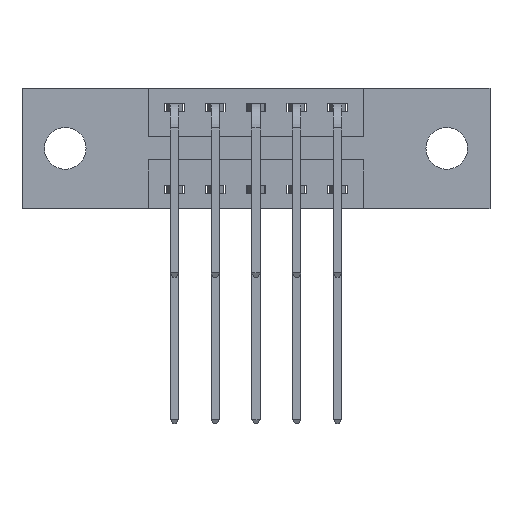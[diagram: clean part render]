
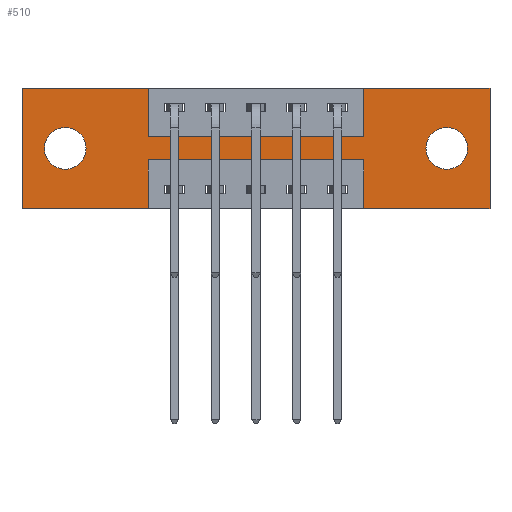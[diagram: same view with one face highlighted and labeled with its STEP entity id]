
A CAD part, front view. The second image highlights one B-rep face of the part: STEP entity #510.
In plain terms, the highlighted planar face has unit normal (0, -1, 0).
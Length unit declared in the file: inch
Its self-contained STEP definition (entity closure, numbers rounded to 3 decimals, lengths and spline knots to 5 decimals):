
#26 = LINE ( 'NONE', #8358, #9534 ) ;
#68 = VECTOR ( 'NONE', #4947, 39.37008 ) ;
#191 = LINE ( 'NONE', #3979, #1855 ) ;
#218 = VECTOR ( 'NONE', #2254, 39.37008 ) ;
#464 = ORIENTED_EDGE ( 'NONE', *, *, #4094, .T. ) ;
#473 = AXIS2_PLACEMENT_3D ( 'NONE', #3910, #2946, #4568 ) ;
#510 = ADVANCED_FACE ( 'NONE', ( #6806, #5420, #1509 ), #10048, .T. ) ;
#543 = CARTESIAN_POINT ( 'NONE',  ( 0., 0., 0. ) ) ;
#584 = VERTEX_POINT ( 'NONE', #8944 ) ;
#598 = ORIENTED_EDGE ( 'NONE', *, *, #5182, .F. ) ;
#751 = DIRECTION ( 'NONE',  ( 0., 0., 1. ) ) ;
#827 = DIRECTION ( 'NONE',  ( -1., 0., 0. ) ) ;
#832 = ORIENTED_EDGE ( 'NONE', *, *, #1442, .F. ) ;
#926 = EDGE_CURVE ( 'NONE', #9453, #1668, #6404, .T. ) ;
#937 = VERTEX_POINT ( 'NONE', #5608 ) ;
#1012 = CARTESIAN_POINT ( 'NONE',  ( 0., 0., -0.37 ) ) ;
#1016 = AXIS2_PLACEMENT_3D ( 'NONE', #6618, #3431, #8939 ) ;
#1019 = ORIENTED_EDGE ( 'NONE', *, *, #2930, .F. ) ;
#1284 = CARTESIAN_POINT ( 'NONE',  ( 1.0475, 0., -0.37 ) ) ;
#1317 = CARTESIAN_POINT ( 'NONE',  ( 0.3875, 0., -0.15 ) ) ;
#1340 = CARTESIAN_POINT ( 'NONE',  ( 1.435, 0., 0. ) ) ;
#1442 = EDGE_CURVE ( 'NONE', #2515, #5428, #1821, .T. ) ;
#1456 = CARTESIAN_POINT ( 'NONE',  ( 1.3025, 0., -0.121 ) ) ;
#1509 = FACE_OUTER_BOUND ( 'NONE', #7575, .T. ) ;
#1668 = VERTEX_POINT ( 'NONE', #4661 ) ;
#1685 = VECTOR ( 'NONE', #751, 39.37008 ) ;
#1821 = LINE ( 'NONE', #5022, #8274 ) ;
#1849 = EDGE_CURVE ( 'NONE', #937, #10002, #4997, .T. ) ;
#1855 = VECTOR ( 'NONE', #4848, 39.37008 ) ;
#1958 = LINE ( 'NONE', #6720, #8975 ) ;
#2009 = DIRECTION ( 'NONE',  ( -1., 0., 0. ) ) ;
#2055 = ORIENTED_EDGE ( 'NONE', *, *, #8290, .T. ) ;
#2098 = VERTEX_POINT ( 'NONE', #3511 ) ;
#2107 = VERTEX_POINT ( 'NONE', #9120 ) ;
#2242 = CIRCLE ( 'NONE', #6442, 0.064 ) ;
#2252 = ORIENTED_EDGE ( 'NONE', *, *, #926, .F. ) ;
#2254 = DIRECTION ( 'NONE',  ( 1., 0., 0. ) ) ;
#2317 = ORIENTED_EDGE ( 'NONE', *, *, #5164, .F. ) ;
#2396 = AXIS2_PLACEMENT_3D ( 'NONE', #2886, #8105, #2783 ) ;
#2399 = ORIENTED_EDGE ( 'NONE', *, *, #5501, .T. ) ;
#2515 = VERTEX_POINT ( 'NONE', #3688 ) ;
#2653 = LINE ( 'NONE', #4118, #8060 ) ;
#2767 = CARTESIAN_POINT ( 'NONE',  ( 1.435, 0., 0. ) ) ;
#2770 = EDGE_CURVE ( 'NONE', #4316, #9453, #26, .T. ) ;
#2783 = DIRECTION ( 'NONE',  ( 0., 0., -1. ) ) ;
#2833 = CARTESIAN_POINT ( 'NONE',  ( 0., 0., -0.37 ) ) ;
#2886 = CARTESIAN_POINT ( 'NONE',  ( 1.3025, 0., -0.185 ) ) ;
#2930 = EDGE_CURVE ( 'NONE', #2098, #3526, #6252, .T. ) ;
#2946 = DIRECTION ( 'NONE',  ( 0., -1., 0. ) ) ;
#2958 = CARTESIAN_POINT ( 'NONE',  ( 1.0475, 0., -0.22 ) ) ;
#3173 = VECTOR ( 'NONE', #9866, 39.37008 ) ;
#3331 = EDGE_LOOP ( 'NONE', ( #5442, #464 ) ) ;
#3388 = CARTESIAN_POINT ( 'NONE',  ( 0.3875, 0., -0.37 ) ) ;
#3414 = DIRECTION ( 'NONE',  ( 1., 0., 0. ) ) ;
#3431 = DIRECTION ( 'NONE',  ( 0., 1., 0. ) ) ;
#3483 = AXIS2_PLACEMENT_3D ( 'NONE', #5290, #8271, #9079 ) ;
#3511 = CARTESIAN_POINT ( 'NONE',  ( 1.435, 0., -0.37 ) ) ;
#3526 = VERTEX_POINT ( 'NONE', #1284 ) ;
#3663 = VECTOR ( 'NONE', #3670, 39.37008 ) ;
#3670 = DIRECTION ( 'NONE',  ( 1., 0., 0. ) ) ;
#3688 = CARTESIAN_POINT ( 'NONE',  ( 0.3875, 0., 0. ) ) ;
#3696 = EDGE_LOOP ( 'NONE', ( #2055, #2399 ) ) ;
#3824 = ORIENTED_EDGE ( 'NONE', *, *, #6346, .F. ) ;
#3896 = ORIENTED_EDGE ( 'NONE', *, *, #9078, .F. ) ;
#3910 = CARTESIAN_POINT ( 'NONE',  ( 0., 0., -0.37 ) ) ;
#3973 = DIRECTION ( 'NONE',  ( 0., 0., -1. ) ) ;
#3979 = CARTESIAN_POINT ( 'NONE',  ( 0.3875, 0., -0.37 ) ) ;
#4014 = CARTESIAN_POINT ( 'NONE',  ( 1.0475, 0., -0.15 ) ) ;
#4094 = EDGE_CURVE ( 'NONE', #2107, #6915, #2242, .T. ) ;
#4118 = CARTESIAN_POINT ( 'NONE',  ( 0., 0., 0. ) ) ;
#4181 = VERTEX_POINT ( 'NONE', #1456 ) ;
#4316 = VERTEX_POINT ( 'NONE', #3388 ) ;
#4467 = CIRCLE ( 'NONE', #1016, 0.064 ) ;
#4568 = DIRECTION ( 'NONE',  ( 0., 0., -1. ) ) ;
#4592 = LINE ( 'NONE', #8286, #3173 ) ;
#4608 = CARTESIAN_POINT ( 'NONE',  ( 0.1325, 0., -0.185 ) ) ;
#4661 = CARTESIAN_POINT ( 'NONE',  ( 0., 0., 0. ) ) ;
#4848 = DIRECTION ( 'NONE',  ( 0., 0., -1. ) ) ;
#4863 = EDGE_CURVE ( 'NONE', #6915, #2107, #4467, .T. ) ;
#4915 = EDGE_CURVE ( 'NONE', #10002, #2098, #9708, .T. ) ;
#4947 = DIRECTION ( 'NONE',  ( -1., 0., 0. ) ) ;
#4997 = LINE ( 'NONE', #543, #3663 ) ;
#5022 = CARTESIAN_POINT ( 'NONE',  ( 0.3875, 0., 0. ) ) ;
#5164 = EDGE_CURVE ( 'NONE', #3526, #6762, #6351, .T. ) ;
#5182 = EDGE_CURVE ( 'NONE', #8281, #4316, #191, .T. ) ;
#5290 = CARTESIAN_POINT ( 'NONE',  ( 1.3025, 0., -0.185 ) ) ;
#5329 = DIRECTION ( 'NONE',  ( 0., 0., 1. ) ) ;
#5420 = FACE_BOUND ( 'NONE', #3331, .T. ) ;
#5428 = VERTEX_POINT ( 'NONE', #1317 ) ;
#5442 = ORIENTED_EDGE ( 'NONE', *, *, #4863, .T. ) ;
#5501 = EDGE_CURVE ( 'NONE', #584, #4181, #7851, .T. ) ;
#5608 = CARTESIAN_POINT ( 'NONE',  ( 1.0475, 0., 0. ) ) ;
#5743 = CARTESIAN_POINT ( 'NONE',  ( 0., 0., 0. ) ) ;
#6107 = ORIENTED_EDGE ( 'NONE', *, *, #4915, .F. ) ;
#6112 = DIRECTION ( 'NONE',  ( 0., 1., 0. ) ) ;
#6235 = EDGE_CURVE ( 'NONE', #6762, #8281, #1958, .T. ) ;
#6252 = LINE ( 'NONE', #1012, #68 ) ;
#6346 = EDGE_CURVE ( 'NONE', #8073, #937, #4592, .T. ) ;
#6351 = LINE ( 'NONE', #8677, #1685 ) ;
#6404 = LINE ( 'NONE', #5743, #6845 ) ;
#6442 = AXIS2_PLACEMENT_3D ( 'NONE', #4608, #6112, #5329 ) ;
#6618 = CARTESIAN_POINT ( 'NONE',  ( 0.1325, 0., -0.185 ) ) ;
#6636 = CARTESIAN_POINT ( 'NONE',  ( 0.3875, 0., -0.22 ) ) ;
#6702 = EDGE_CURVE ( 'NONE', #5428, #8073, #7725, .T. ) ;
#6707 = VECTOR ( 'NONE', #9659, 39.37008 ) ;
#6720 = CARTESIAN_POINT ( 'NONE',  ( 0.3875, 0., -0.22 ) ) ;
#6762 = VERTEX_POINT ( 'NONE', #2958 ) ;
#6806 = FACE_BOUND ( 'NONE', #3696, .T. ) ;
#6827 = ORIENTED_EDGE ( 'NONE', *, *, #6235, .F. ) ;
#6845 = VECTOR ( 'NONE', #8828, 39.37008 ) ;
#6915 = VERTEX_POINT ( 'NONE', #9531 ) ;
#7575 = EDGE_LOOP ( 'NONE', ( #598, #6827, #2317, #1019, #6107, #9064, #3824, #7966, #832, #3896, #2252, #8906 ) ) ;
#7631 = CARTESIAN_POINT ( 'NONE',  ( 0.3875, 0., -0.15 ) ) ;
#7725 = LINE ( 'NONE', #7631, #218 ) ;
#7747 = CIRCLE ( 'NONE', #2396, 0.064 ) ;
#7851 = CIRCLE ( 'NONE', #3483, 0.064 ) ;
#7966 = ORIENTED_EDGE ( 'NONE', *, *, #6702, .F. ) ;
#8060 = VECTOR ( 'NONE', #3414, 39.37008 ) ;
#8073 = VERTEX_POINT ( 'NONE', #4014 ) ;
#8105 = DIRECTION ( 'NONE',  ( 0., 1., 0. ) ) ;
#8271 = DIRECTION ( 'NONE',  ( 0., 1., 0. ) ) ;
#8274 = VECTOR ( 'NONE', #3973, 39.37008 ) ;
#8281 = VERTEX_POINT ( 'NONE', #6636 ) ;
#8286 = CARTESIAN_POINT ( 'NONE',  ( 1.0475, 0., 0. ) ) ;
#8290 = EDGE_CURVE ( 'NONE', #4181, #584, #7747, .T. ) ;
#8358 = CARTESIAN_POINT ( 'NONE',  ( 0., 0., -0.37 ) ) ;
#8677 = CARTESIAN_POINT ( 'NONE',  ( 1.0475, 0., -0.37 ) ) ;
#8828 = DIRECTION ( 'NONE',  ( 0., 0., 1. ) ) ;
#8906 = ORIENTED_EDGE ( 'NONE', *, *, #2770, .F. ) ;
#8939 = DIRECTION ( 'NONE',  ( 0., 0., 1. ) ) ;
#8944 = CARTESIAN_POINT ( 'NONE',  ( 1.3025, 0., -0.249 ) ) ;
#8975 = VECTOR ( 'NONE', #2009, 39.37008 ) ;
#9064 = ORIENTED_EDGE ( 'NONE', *, *, #1849, .F. ) ;
#9078 = EDGE_CURVE ( 'NONE', #1668, #2515, #2653, .T. ) ;
#9079 = DIRECTION ( 'NONE',  ( 0., 0., -1. ) ) ;
#9120 = CARTESIAN_POINT ( 'NONE',  ( 0.1325, 0., -0.249 ) ) ;
#9453 = VERTEX_POINT ( 'NONE', #2833 ) ;
#9531 = CARTESIAN_POINT ( 'NONE',  ( 0.1325, 0., -0.121 ) ) ;
#9534 = VECTOR ( 'NONE', #827, 39.37008 ) ;
#9659 = DIRECTION ( 'NONE',  ( 0., 0., -1. ) ) ;
#9708 = LINE ( 'NONE', #2767, #6707 ) ;
#9866 = DIRECTION ( 'NONE',  ( 0., 0., 1. ) ) ;
#10002 = VERTEX_POINT ( 'NONE', #1340 ) ;
#10048 = PLANE ( 'NONE',  #473 ) ;
